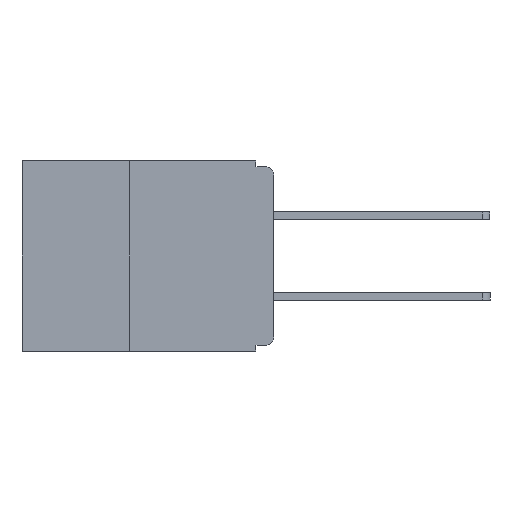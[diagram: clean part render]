
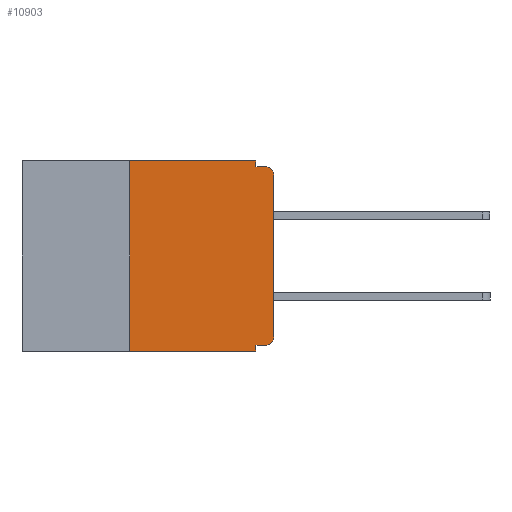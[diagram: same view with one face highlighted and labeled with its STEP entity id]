
A CAD part, left-side view. The second image highlights one B-rep face of the part: STEP entity #10903.
In plain terms, the highlighted planar face has unit normal (-1, 0, 0).
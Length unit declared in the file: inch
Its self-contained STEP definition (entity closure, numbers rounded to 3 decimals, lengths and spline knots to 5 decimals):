
#41 = CARTESIAN_POINT ( 'NONE',  ( 0., 0.015, -0.01 ) ) ;
#81 = VECTOR ( 'NONE', #10488, 39.37008 ) ;
#146 = VECTOR ( 'NONE', #2367, 39.37008 ) ;
#321 = ORIENTED_EDGE ( 'NONE', *, *, #21902, .F. ) ;
#523 = EDGE_CURVE ( 'NONE', #5151, #1763, #4886, .T. ) ;
#639 = DIRECTION ( 'NONE',  ( 0., 0., 1. ) ) ;
#1322 = CARTESIAN_POINT ( 'NONE',  ( 0., 0.015, -0.32 ) ) ;
#1441 = ORIENTED_EDGE ( 'NONE', *, *, #18201, .T. ) ;
#1763 = VERTEX_POINT ( 'NONE', #3387 ) ;
#2230 = EDGE_CURVE ( 'NONE', #9469, #19800, #2491, .T. ) ;
#2348 = CARTESIAN_POINT ( 'NONE',  ( 0., 0.031, -0.33 ) ) ;
#2367 = DIRECTION ( 'NONE',  ( 0., 1., 0. ) ) ;
#2491 = LINE ( 'NONE', #9423, #6930 ) ;
#3387 = CARTESIAN_POINT ( 'NONE',  ( 0., 0.25, 0. ) ) ;
#3646 = VERTEX_POINT ( 'NONE', #15873 ) ;
#4238 = VERTEX_POINT ( 'NONE', #4540 ) ;
#4367 = DIRECTION ( 'NONE',  ( 0., 0., -1. ) ) ;
#4428 = CARTESIAN_POINT ( 'NONE',  ( 0., 0., 0. ) ) ;
#4540 = CARTESIAN_POINT ( 'NONE',  ( 0., 0., -0.025 ) ) ;
#4886 = LINE ( 'NONE', #10114, #14812 ) ;
#5000 = ORIENTED_EDGE ( 'NONE', *, *, #2230, .F. ) ;
#5024 = EDGE_LOOP ( 'NONE', ( #1441, #21799, #8233, #5000, #16618, #13548, #14098, #19519, #321, #10348 ) ) ;
#5151 = VERTEX_POINT ( 'NONE', #14461 ) ;
#5864 = DIRECTION ( 'NONE',  ( 0., -1., 0. ) ) ;
#6034 = EDGE_CURVE ( 'NONE', #1763, #9469, #8228, .T. ) ;
#6700 = VERTEX_POINT ( 'NONE', #2348 ) ;
#6809 = DIRECTION ( 'NONE',  ( -1., 0., 0. ) ) ;
#6930 = VECTOR ( 'NONE', #4367, 39.37008 ) ;
#7175 = VERTEX_POINT ( 'NONE', #41 ) ;
#8228 = LINE ( 'NONE', #17132, #22359 ) ;
#8233 = ORIENTED_EDGE ( 'NONE', *, *, #15659, .F. ) ;
#8363 = CARTESIAN_POINT ( 'NONE',  ( 0., 0.031, -0.32 ) ) ;
#8413 = VECTOR ( 'NONE', #5864, 39.37008 ) ;
#8599 = CARTESIAN_POINT ( 'NONE',  ( 0., 0.031, -0.33 ) ) ;
#9423 = CARTESIAN_POINT ( 'NONE',  ( 0., 0.031, 0. ) ) ;
#9469 = VERTEX_POINT ( 'NONE', #20392 ) ;
#9821 = EDGE_CURVE ( 'NONE', #4238, #7175, #15600, .T. ) ;
#9868 = PLANE ( 'NONE',  #20473 ) ;
#10059 = CIRCLE ( 'NONE', #11957, 0.015 ) ;
#10114 = CARTESIAN_POINT ( 'NONE',  ( 0., 0.25, -0.33 ) ) ;
#10312 = DIRECTION ( 'NONE',  ( -1., 0., 0. ) ) ;
#10348 = ORIENTED_EDGE ( 'NONE', *, *, #17686, .T. ) ;
#10381 = FACE_OUTER_BOUND ( 'NONE', #5024, .T. ) ;
#10488 = DIRECTION ( 'NONE',  ( 0., 0., -1. ) ) ;
#10903 = ADVANCED_FACE ( 'NONE', ( #10381 ), #9868, .F. ) ;
#11295 = VECTOR ( 'NONE', #15088, 39.37008 ) ;
#11733 = DIRECTION ( 'NONE',  ( 0., 0., -1. ) ) ;
#11957 = AXIS2_PLACEMENT_3D ( 'NONE', #21297, #10312, #23133 ) ;
#12816 = LINE ( 'NONE', #20667, #8413 ) ;
#13237 = LINE ( 'NONE', #4428, #18081 ) ;
#13290 = CARTESIAN_POINT ( 'NONE',  ( 0., 0., -0.01 ) ) ;
#13310 = DIRECTION ( 'NONE',  ( 0., 0., 1. ) ) ;
#13548 = ORIENTED_EDGE ( 'NONE', *, *, #523, .F. ) ;
#14098 = ORIENTED_EDGE ( 'NONE', *, *, #14516, .T. ) ;
#14461 = CARTESIAN_POINT ( 'NONE',  ( 0., 0.25, -0.33 ) ) ;
#14516 = EDGE_CURVE ( 'NONE', #5151, #6700, #12816, .T. ) ;
#14812 = VECTOR ( 'NONE', #13310, 39.37008 ) ;
#14885 = VERTEX_POINT ( 'NONE', #1322 ) ;
#14987 = LINE ( 'NONE', #8599, #81 ) ;
#15053 = LINE ( 'NONE', #20885, #146 ) ;
#15088 = DIRECTION ( 'NONE',  ( 0., -1., 0. ) ) ;
#15600 = CIRCLE ( 'NONE', #19842, 0.015 ) ;
#15659 = EDGE_CURVE ( 'NONE', #19800, #7175, #21623, .T. ) ;
#15873 = CARTESIAN_POINT ( 'NONE',  ( 0., 0., -0.305 ) ) ;
#16618 = ORIENTED_EDGE ( 'NONE', *, *, #6034, .F. ) ;
#17132 = CARTESIAN_POINT ( 'NONE',  ( 0., 0.437, 0. ) ) ;
#17156 = CARTESIAN_POINT ( 'NONE',  ( 0., 0.437, 0. ) ) ;
#17686 = EDGE_CURVE ( 'NONE', #14885, #3646, #10059, .T. ) ;
#17903 = CARTESIAN_POINT ( 'NONE',  ( 0., 0.015, -0.025 ) ) ;
#18011 = CARTESIAN_POINT ( 'NONE',  ( 0., 0.031, -0.01 ) ) ;
#18081 = VECTOR ( 'NONE', #639, 39.37008 ) ;
#18201 = EDGE_CURVE ( 'NONE', #3646, #4238, #13237, .T. ) ;
#18985 = DIRECTION ( 'NONE',  ( 0., -1., 0. ) ) ;
#19519 = ORIENTED_EDGE ( 'NONE', *, *, #23257, .F. ) ;
#19742 = DIRECTION ( 'NONE',  ( 0., 0., -1. ) ) ;
#19800 = VERTEX_POINT ( 'NONE', #18011 ) ;
#19842 = AXIS2_PLACEMENT_3D ( 'NONE', #17903, #6809, #19742 ) ;
#20392 = CARTESIAN_POINT ( 'NONE',  ( 0., 0.031, 0. ) ) ;
#20473 = AXIS2_PLACEMENT_3D ( 'NONE', #17156, #22691, #11733 ) ;
#20667 = CARTESIAN_POINT ( 'NONE',  ( 0., 0.437, -0.33 ) ) ;
#20885 = CARTESIAN_POINT ( 'NONE',  ( 0., 0., -0.32 ) ) ;
#21297 = CARTESIAN_POINT ( 'NONE',  ( 0., 0.015, -0.305 ) ) ;
#21623 = LINE ( 'NONE', #13290, #11295 ) ;
#21799 = ORIENTED_EDGE ( 'NONE', *, *, #9821, .T. ) ;
#21902 = EDGE_CURVE ( 'NONE', #14885, #22716, #15053, .T. ) ;
#22359 = VECTOR ( 'NONE', #18985, 39.37008 ) ;
#22691 = DIRECTION ( 'NONE',  ( 1., 0., 0. ) ) ;
#22716 = VERTEX_POINT ( 'NONE', #8363 ) ;
#23133 = DIRECTION ( 'NONE',  ( 0., 0., -1. ) ) ;
#23257 = EDGE_CURVE ( 'NONE', #22716, #6700, #14987, .T. ) ;
